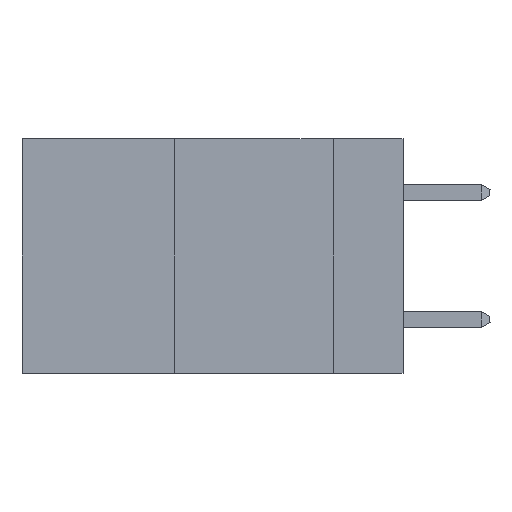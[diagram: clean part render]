
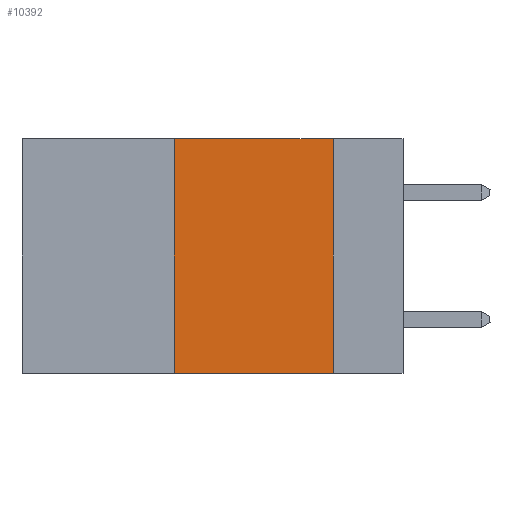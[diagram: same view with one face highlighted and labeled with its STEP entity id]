
A CAD part, left-side view. The second image highlights one B-rep face of the part: STEP entity #10392.
In plain terms, the highlighted planar face has unit normal (-1, 0, 0).
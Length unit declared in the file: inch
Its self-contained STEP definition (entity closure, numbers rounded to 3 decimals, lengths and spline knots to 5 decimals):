
#1109 = CARTESIAN_POINT ( 'NONE',  ( 0., 0.36, -0.37 ) ) ;
#1174 = LINE ( 'NONE', #2443, #5644 ) ;
#1710 = VERTEX_POINT ( 'NONE', #1109 ) ;
#1844 = CARTESIAN_POINT ( 'NONE',  ( 0., 0.11, -0.37 ) ) ;
#2443 = CARTESIAN_POINT ( 'NONE',  ( 0., 0.6, 0. ) ) ;
#4121 = DIRECTION ( 'NONE',  ( 0., -1., 0. ) ) ;
#4264 = CARTESIAN_POINT ( 'NONE',  ( 0., 0.11, 0. ) ) ;
#4731 = ORIENTED_EDGE ( 'NONE', *, *, #14190, .F. ) ;
#5070 = VERTEX_POINT ( 'NONE', #4264 ) ;
#5505 = EDGE_LOOP ( 'NONE', ( #16911, #4731, #14621, #11161 ) ) ;
#5644 = VECTOR ( 'NONE', #14867, 39.37008 ) ;
#6164 = CARTESIAN_POINT ( 'NONE',  ( 0., 0.36, 0. ) ) ;
#6184 = EDGE_CURVE ( 'NONE', #1710, #6263, #9842, .T. ) ;
#6263 = VERTEX_POINT ( 'NONE', #1844 ) ;
#7815 = AXIS2_PLACEMENT_3D ( 'NONE', #13764, #16398, #11098 ) ;
#8283 = EDGE_CURVE ( 'NONE', #5070, #6263, #12314, .T. ) ;
#8466 = VECTOR ( 'NONE', #16986, 39.37008 ) ;
#9842 = LINE ( 'NONE', #16198, #13650 ) ;
#10125 = LINE ( 'NONE', #6164, #8466 ) ;
#10143 = CARTESIAN_POINT ( 'NONE',  ( 0., 0.11, 0. ) ) ;
#10392 = ADVANCED_FACE ( 'NONE', ( #15077 ), #14936, .F. ) ;
#11098 = DIRECTION ( 'NONE',  ( 0., 0., -1. ) ) ;
#11161 = ORIENTED_EDGE ( 'NONE', *, *, #6184, .T. ) ;
#11786 = EDGE_CURVE ( 'NONE', #1710, #13045, #10125, .T. ) ;
#12314 = LINE ( 'NONE', #10143, #15062 ) ;
#13045 = VERTEX_POINT ( 'NONE', #15294 ) ;
#13650 = VECTOR ( 'NONE', #4121, 39.37008 ) ;
#13764 = CARTESIAN_POINT ( 'NONE',  ( 0., 0.6, 0. ) ) ;
#14190 = EDGE_CURVE ( 'NONE', #13045, #5070, #1174, .T. ) ;
#14239 = DIRECTION ( 'NONE',  ( 0., 0., -1. ) ) ;
#14621 = ORIENTED_EDGE ( 'NONE', *, *, #11786, .F. ) ;
#14867 = DIRECTION ( 'NONE',  ( 0., -1., 0. ) ) ;
#14936 = PLANE ( 'NONE',  #7815 ) ;
#15062 = VECTOR ( 'NONE', #14239, 39.37008 ) ;
#15077 = FACE_OUTER_BOUND ( 'NONE', #5505, .T. ) ;
#15294 = CARTESIAN_POINT ( 'NONE',  ( 0., 0.36, 0. ) ) ;
#16198 = CARTESIAN_POINT ( 'NONE',  ( 0., 0.6, -0.37 ) ) ;
#16398 = DIRECTION ( 'NONE',  ( 1., 0., 0. ) ) ;
#16911 = ORIENTED_EDGE ( 'NONE', *, *, #8283, .F. ) ;
#16986 = DIRECTION ( 'NONE',  ( 0., 0., 1. ) ) ;
